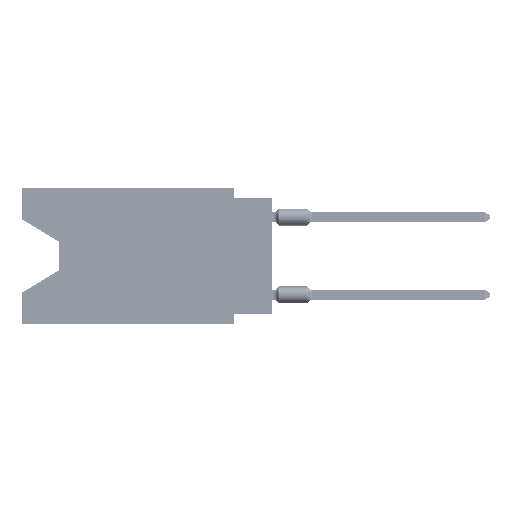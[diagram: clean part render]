
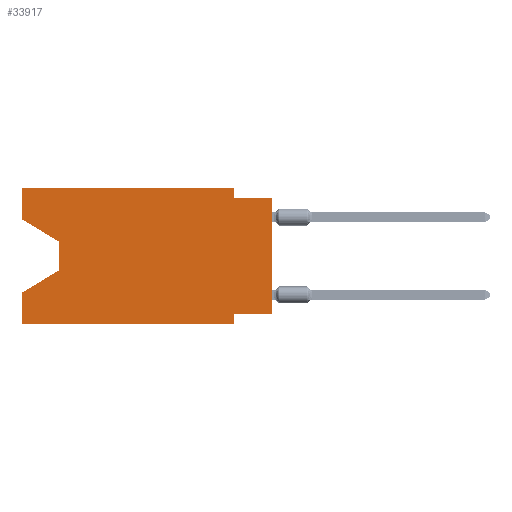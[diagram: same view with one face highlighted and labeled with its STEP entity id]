
A CAD part, left-side view. The second image highlights one B-rep face of the part: STEP entity #33917.
In plain terms, the highlighted planar face has unit normal (-1, 0, 0).
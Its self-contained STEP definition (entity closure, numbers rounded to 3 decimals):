
#258 = CARTESIAN_POINT ( 'NONE',  ( 0., 2.54, -8.255 ) ) ;
#442 = DIRECTION ( 'NONE',  ( 0., -1., 0. ) ) ;
#624 = VERTEX_POINT ( 'NONE', #65319 ) ;
#880 = ORIENTED_EDGE ( 'NONE', *, *, #69108, .T. ) ;
#3292 = CARTESIAN_POINT ( 'NONE',  ( 0., 2.54, -8.89 ) ) ;
#3803 = DIRECTION ( 'NONE',  ( 0., 0., -1. ) ) ;
#7338 = LINE ( 'NONE', #38720, #51485 ) ;
#7685 = CARTESIAN_POINT ( 'NONE',  ( 0., 2.54, 0. ) ) ;
#8121 = VECTOR ( 'NONE', #50193, 1000. ) ;
#9164 = VECTOR ( 'NONE', #34258, 1000. ) ;
#10226 = EDGE_CURVE ( 'NONE', #92339, #80978, #47638, .T. ) ;
#12935 = LINE ( 'NONE', #98814, #50747 ) ;
#13196 = EDGE_CURVE ( 'NONE', #42418, #91703, #79119, .T. ) ;
#14126 = VERTEX_POINT ( 'NONE', #27790 ) ;
#18486 = ORIENTED_EDGE ( 'NONE', *, *, #23615, .F. ) ;
#21002 = CARTESIAN_POINT ( 'NONE',  ( 0., 0., -8.255 ) ) ;
#23615 = EDGE_CURVE ( 'NONE', #48483, #36308, #51510, .T. ) ;
#24229 = VECTOR ( 'NONE', #46702, 1000. ) ;
#26094 = ORIENTED_EDGE ( 'NONE', *, *, #91469, .F. ) ;
#26203 = EDGE_LOOP ( 'NONE', ( #28582, #39479, #88473, #95296, #67770, #26094, #18486, #880, #97865, #88073, #34528, #84427 ) ) ;
#26567 = VECTOR ( 'NONE', #60113, 1000. ) ;
#27790 = CARTESIAN_POINT ( 'NONE',  ( 0., 13.97, -3.505 ) ) ;
#28294 = EDGE_CURVE ( 'NONE', #624, #92973, #62261, .T. ) ;
#28582 = ORIENTED_EDGE ( 'NONE', *, *, #98113, .T. ) ;
#28759 = CARTESIAN_POINT ( 'NONE',  ( 0., 16.383, -2.038 ) ) ;
#31803 = CARTESIAN_POINT ( 'NONE',  ( 0., 16.383, 0. ) ) ;
#32475 = DIRECTION ( 'NONE',  ( 0., 0., 1. ) ) ;
#32743 = VECTOR ( 'NONE', #3803, 1000. ) ;
#32937 = VECTOR ( 'NONE', #442, 1000. ) ;
#33917 = ADVANCED_FACE ( 'NONE', ( #38744 ), #92251, .F. ) ;
#34258 = DIRECTION ( 'NONE',  ( 0., -1., 0. ) ) ;
#34528 = ORIENTED_EDGE ( 'NONE', *, *, #13196, .F. ) ;
#36308 = VERTEX_POINT ( 'NONE', #258 ) ;
#36324 = VECTOR ( 'NONE', #32475, 1000. ) ;
#38261 = EDGE_CURVE ( 'NONE', #91703, #93003, #12935, .T. ) ;
#38720 = CARTESIAN_POINT ( 'NONE',  ( 0., 0., 0. ) ) ;
#38744 = FACE_OUTER_BOUND ( 'NONE', #26203, .T. ) ;
#39479 = ORIENTED_EDGE ( 'NONE', *, *, #76384, .T. ) ;
#40183 = CARTESIAN_POINT ( 'NONE',  ( 0., 16.383, 0. ) ) ;
#41319 = DIRECTION ( 'NONE',  ( 0., 1., 0. ) ) ;
#41473 = CARTESIAN_POINT ( 'NONE',  ( 0., 0., -0.635 ) ) ;
#41498 = CARTESIAN_POINT ( 'NONE',  ( 0., 13.97, -3.505 ) ) ;
#42418 = VERTEX_POINT ( 'NONE', #68797 ) ;
#44199 = LINE ( 'NONE', #28759, #26567 ) ;
#44306 = DIRECTION ( 'NONE',  ( 0., 0., -1. ) ) ;
#44635 = VECTOR ( 'NONE', #61758, 1000. ) ;
#46636 = CARTESIAN_POINT ( 'NONE',  ( 0., 16.383, -2.038 ) ) ;
#46702 = DIRECTION ( 'NONE',  ( 0., 0., 1. ) ) ;
#46735 = CARTESIAN_POINT ( 'NONE',  ( 0., 16.383, 0. ) ) ;
#47027 = VECTOR ( 'NONE', #41319, 1000. ) ;
#47638 = LINE ( 'NONE', #64088, #64719 ) ;
#48483 = VERTEX_POINT ( 'NONE', #21002 ) ;
#48972 = CARTESIAN_POINT ( 'NONE',  ( 0., 16.383, -6.852 ) ) ;
#50193 = DIRECTION ( 'NONE',  ( 0., 0., -1. ) ) ;
#50213 = CARTESIAN_POINT ( 'NONE',  ( 0., 16.383, -8.89 ) ) ;
#50747 = VECTOR ( 'NONE', #44306, 1000. ) ;
#51485 = VECTOR ( 'NONE', #70062, 1000. ) ;
#51510 = LINE ( 'NONE', #82879, #47027 ) ;
#52743 = EDGE_CURVE ( 'NONE', #92339, #92973, #69977, .T. ) ;
#55854 = DIRECTION ( 'NONE',  ( 0., -1., 0. ) ) ;
#56308 = EDGE_CURVE ( 'NONE', #67398, #42418, #60229, .T. ) ;
#60113 = DIRECTION ( 'NONE',  ( 0., -0.855, -0.519 ) ) ;
#60229 = LINE ( 'NONE', #31803, #24229 ) ;
#61758 = DIRECTION ( 'NONE',  ( 0., 0.855, -0.519 ) ) ;
#62261 = LINE ( 'NONE', #93644, #44635 ) ;
#64088 = CARTESIAN_POINT ( 'NONE',  ( 0., 16.383, -8.89 ) ) ;
#64719 = VECTOR ( 'NONE', #55854, 1000. ) ;
#65319 = CARTESIAN_POINT ( 'NONE',  ( 0., 13.97, -5.385 ) ) ;
#66518 = LINE ( 'NONE', #3292, #32743 ) ;
#67398 = VERTEX_POINT ( 'NONE', #46636 ) ;
#67770 = ORIENTED_EDGE ( 'NONE', *, *, #10226, .T. ) ;
#68797 = CARTESIAN_POINT ( 'NONE',  ( 0., 16.383, 0. ) ) ;
#69108 = EDGE_CURVE ( 'NONE', #48483, #81949, #7338, .T. ) ;
#69977 = LINE ( 'NONE', #40183, #36324 ) ;
#70062 = DIRECTION ( 'NONE',  ( 0., 0., 1. ) ) ;
#70593 = DIRECTION ( 'NONE',  ( 0., 0., -1. ) ) ;
#74155 = CARTESIAN_POINT ( 'NONE',  ( 0., 2.54, -8.89 ) ) ;
#76384 = EDGE_CURVE ( 'NONE', #14126, #624, #88285, .T. ) ;
#76640 = AXIS2_PLACEMENT_3D ( 'NONE', #93254, #92754, #70593 ) ;
#79119 = LINE ( 'NONE', #46735, #32937 ) ;
#80978 = VERTEX_POINT ( 'NONE', #74155 ) ;
#81949 = VERTEX_POINT ( 'NONE', #95324 ) ;
#82879 = CARTESIAN_POINT ( 'NONE',  ( 0., 0., -8.255 ) ) ;
#84427 = ORIENTED_EDGE ( 'NONE', *, *, #56308, .F. ) ;
#87622 = EDGE_CURVE ( 'NONE', #93003, #81949, #95466, .T. ) ;
#88073 = ORIENTED_EDGE ( 'NONE', *, *, #38261, .F. ) ;
#88285 = LINE ( 'NONE', #41498, #8121 ) ;
#88473 = ORIENTED_EDGE ( 'NONE', *, *, #28294, .T. ) ;
#91469 = EDGE_CURVE ( 'NONE', #36308, #80978, #66518, .T. ) ;
#91703 = VERTEX_POINT ( 'NONE', #7685 ) ;
#92251 = PLANE ( 'NONE',  #76640 ) ;
#92339 = VERTEX_POINT ( 'NONE', #50213 ) ;
#92754 = DIRECTION ( 'NONE',  ( 1., 0., 0. ) ) ;
#92973 = VERTEX_POINT ( 'NONE', #48972 ) ;
#93003 = VERTEX_POINT ( 'NONE', #94227 ) ;
#93254 = CARTESIAN_POINT ( 'NONE',  ( 0., 16.383, 0. ) ) ;
#93644 = CARTESIAN_POINT ( 'NONE',  ( 0., 13.97, -5.385 ) ) ;
#94227 = CARTESIAN_POINT ( 'NONE',  ( 0., 2.54, -0.635 ) ) ;
#95296 = ORIENTED_EDGE ( 'NONE', *, *, #52743, .F. ) ;
#95324 = CARTESIAN_POINT ( 'NONE',  ( 0., 0., -0.635 ) ) ;
#95466 = LINE ( 'NONE', #41473, #9164 ) ;
#97865 = ORIENTED_EDGE ( 'NONE', *, *, #87622, .F. ) ;
#98113 = EDGE_CURVE ( 'NONE', #67398, #14126, #44199, .T. ) ;
#98814 = CARTESIAN_POINT ( 'NONE',  ( 0., 2.54, 0. ) ) ;
